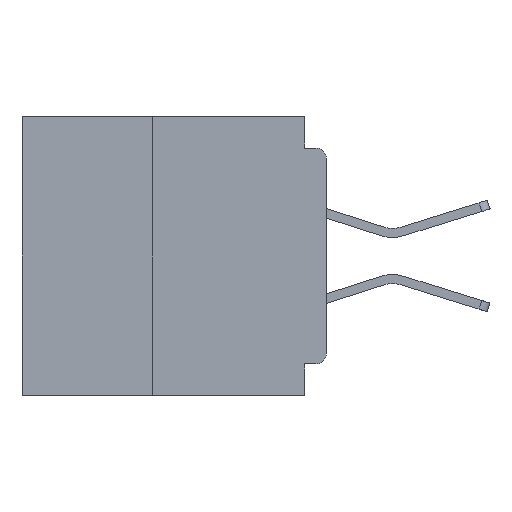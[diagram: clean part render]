
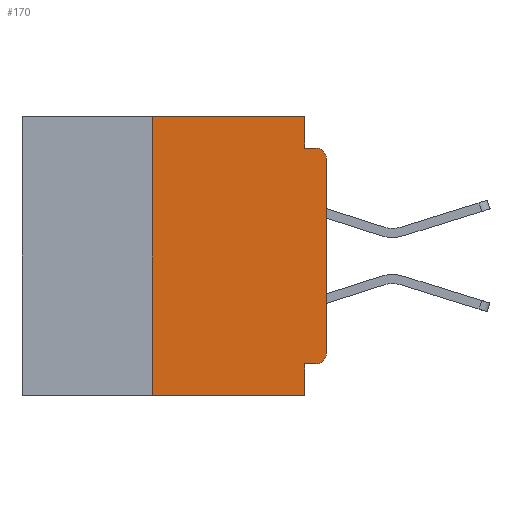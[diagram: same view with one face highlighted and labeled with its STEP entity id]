
A CAD part, left-side view. The second image highlights one B-rep face of the part: STEP entity #170.
In plain terms, the highlighted planar face has unit normal (-1, 0, 0).
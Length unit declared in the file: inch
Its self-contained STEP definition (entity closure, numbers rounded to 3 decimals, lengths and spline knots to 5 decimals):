
#170 = ADVANCED_FACE ( 'NONE', ( #20873 ), #18530, .F. ) ;
#256 = CARTESIAN_POINT ( 'NONE',  ( 0., 0.25, -0.4 ) ) ;
#1623 = CARTESIAN_POINT ( 'NONE',  ( 0., 0., -0.06 ) ) ;
#1699 = VERTEX_POINT ( 'NONE', #38426 ) ;
#2398 = DIRECTION ( 'NONE',  ( 0., 0., -1. ) ) ;
#3183 = CARTESIAN_POINT ( 'NONE',  ( 0., 0., 0. ) ) ;
#3210 = EDGE_CURVE ( 'NONE', #23227, #28093, #6582, .T. ) ;
#4057 = EDGE_CURVE ( 'NONE', #31193, #38917, #17491, .T. ) ;
#4958 = CARTESIAN_POINT ( 'NONE',  ( 0., 0.437, 0. ) ) ;
#5925 = ORIENTED_EDGE ( 'NONE', *, *, #26304, .F. ) ;
#5983 = DIRECTION ( 'NONE',  ( 0., 0., 1. ) ) ;
#6258 = DIRECTION ( 'NONE',  ( 1., 0., 0. ) ) ;
#6339 = CARTESIAN_POINT ( 'NONE',  ( 0., 0.437, 0. ) ) ;
#6582 = LINE ( 'NONE', #3183, #29655 ) ;
#6968 = VECTOR ( 'NONE', #35060, 39.37008 ) ;
#7051 = EDGE_CURVE ( 'NONE', #28093, #1699, #12735, .T. ) ;
#7144 = AXIS2_PLACEMENT_3D ( 'NONE', #6339, #6258, #16620 ) ;
#7480 = DIRECTION ( 'NONE',  ( 0., 0., -1. ) ) ;
#7522 = EDGE_CURVE ( 'NONE', #19861, #24363, #33693, .T. ) ;
#8342 = CARTESIAN_POINT ( 'NONE',  ( 0., 0.25, -0.4 ) ) ;
#9423 = VECTOR ( 'NONE', #36320, 39.37008 ) ;
#10549 = LINE ( 'NONE', #25515, #25561 ) ;
#10840 = CARTESIAN_POINT ( 'NONE',  ( 0., 0.437, -0.4 ) ) ;
#11797 = EDGE_CURVE ( 'NONE', #18014, #23227, #34766, .T. ) ;
#12735 = CIRCLE ( 'NONE', #15233, 0.015 ) ;
#13312 = ORIENTED_EDGE ( 'NONE', *, *, #22354, .F. ) ;
#13706 = ORIENTED_EDGE ( 'NONE', *, *, #3210, .T. ) ;
#13875 = DIRECTION ( 'NONE',  ( -1., 0., 0. ) ) ;
#13972 = LINE ( 'NONE', #25414, #28967 ) ;
#14930 = CARTESIAN_POINT ( 'NONE',  ( 0., 0.25, 0. ) ) ;
#15059 = LINE ( 'NONE', #4958, #6968 ) ;
#15233 = AXIS2_PLACEMENT_3D ( 'NONE', #38491, #20638, #2398 ) ;
#15668 = VECTOR ( 'NONE', #27492, 39.37008 ) ;
#16032 = LINE ( 'NONE', #8342, #30017 ) ;
#16620 = DIRECTION ( 'NONE',  ( 0., 0., -1. ) ) ;
#17491 = LINE ( 'NONE', #36276, #9423 ) ;
#18014 = VERTEX_POINT ( 'NONE', #20208 ) ;
#18530 = PLANE ( 'NONE',  #7144 ) ;
#18863 = VECTOR ( 'NONE', #31731, 39.37008 ) ;
#19861 = VERTEX_POINT ( 'NONE', #256 ) ;
#20208 = CARTESIAN_POINT ( 'NONE',  ( 0., 0.015, -0.355 ) ) ;
#20610 = EDGE_LOOP ( 'NONE', ( #13706, #39123, #5925, #32195, #37987, #13312, #23465, #28019, #34360, #32625 ) ) ;
#20638 = DIRECTION ( 'NONE',  ( -1., 0., 0. ) ) ;
#20873 = FACE_OUTER_BOUND ( 'NONE', #20610, .T. ) ;
#21485 = CARTESIAN_POINT ( 'NONE',  ( 0., 0., -0.045 ) ) ;
#22324 = EDGE_CURVE ( 'NONE', #31907, #31193, #15059, .T. ) ;
#22354 = EDGE_CURVE ( 'NONE', #19861, #31907, #16032, .T. ) ;
#23227 = VERTEX_POINT ( 'NONE', #27350 ) ;
#23465 = ORIENTED_EDGE ( 'NONE', *, *, #7522, .T. ) ;
#23587 = LINE ( 'NONE', #21485, #15668 ) ;
#24363 = VERTEX_POINT ( 'NONE', #32765 ) ;
#25414 = CARTESIAN_POINT ( 'NONE',  ( 0., 0., -0.355 ) ) ;
#25515 = CARTESIAN_POINT ( 'NONE',  ( 0., 0.031, -0.4 ) ) ;
#25561 = VECTOR ( 'NONE', #7480, 39.37008 ) ;
#25778 = CARTESIAN_POINT ( 'NONE',  ( 0., 0.031, -0.355 ) ) ;
#26304 = EDGE_CURVE ( 'NONE', #38917, #1699, #23587, .T. ) ;
#27350 = CARTESIAN_POINT ( 'NONE',  ( 0., 0., -0.34 ) ) ;
#27492 = DIRECTION ( 'NONE',  ( 0., -1., 0. ) ) ;
#28019 = ORIENTED_EDGE ( 'NONE', *, *, #37752, .F. ) ;
#28093 = VERTEX_POINT ( 'NONE', #1623 ) ;
#28422 = DIRECTION ( 'NONE',  ( 0., 1., 0. ) ) ;
#28967 = VECTOR ( 'NONE', #28422, 39.37008 ) ;
#29370 = AXIS2_PLACEMENT_3D ( 'NONE', #31750, #13875, #34764 ) ;
#29655 = VECTOR ( 'NONE', #5983, 39.37008 ) ;
#29796 = CARTESIAN_POINT ( 'NONE',  ( 0., 0.031, -0.045 ) ) ;
#29801 = EDGE_CURVE ( 'NONE', #18014, #37800, #13972, .T. ) ;
#30017 = VECTOR ( 'NONE', #35184, 39.37008 ) ;
#31193 = VERTEX_POINT ( 'NONE', #35490 ) ;
#31731 = DIRECTION ( 'NONE',  ( 0., -1., 0. ) ) ;
#31750 = CARTESIAN_POINT ( 'NONE',  ( 0., 0.015, -0.34 ) ) ;
#31907 = VERTEX_POINT ( 'NONE', #14930 ) ;
#32195 = ORIENTED_EDGE ( 'NONE', *, *, #4057, .F. ) ;
#32625 = ORIENTED_EDGE ( 'NONE', *, *, #11797, .T. ) ;
#32765 = CARTESIAN_POINT ( 'NONE',  ( 0., 0.031, -0.4 ) ) ;
#33693 = LINE ( 'NONE', #10840, #18863 ) ;
#34360 = ORIENTED_EDGE ( 'NONE', *, *, #29801, .F. ) ;
#34764 = DIRECTION ( 'NONE',  ( 0., 0., -1. ) ) ;
#34766 = CIRCLE ( 'NONE', #29370, 0.015 ) ;
#35060 = DIRECTION ( 'NONE',  ( 0., -1., 0. ) ) ;
#35184 = DIRECTION ( 'NONE',  ( 0., 0., 1. ) ) ;
#35490 = CARTESIAN_POINT ( 'NONE',  ( 0., 0.031, 0. ) ) ;
#36276 = CARTESIAN_POINT ( 'NONE',  ( 0., 0.031, 0. ) ) ;
#36320 = DIRECTION ( 'NONE',  ( 0., 0., -1. ) ) ;
#37752 = EDGE_CURVE ( 'NONE', #37800, #24363, #10549, .T. ) ;
#37800 = VERTEX_POINT ( 'NONE', #25778 ) ;
#37987 = ORIENTED_EDGE ( 'NONE', *, *, #22324, .F. ) ;
#38426 = CARTESIAN_POINT ( 'NONE',  ( 0., 0.015, -0.045 ) ) ;
#38491 = CARTESIAN_POINT ( 'NONE',  ( 0., 0.015, -0.06 ) ) ;
#38917 = VERTEX_POINT ( 'NONE', #29796 ) ;
#39123 = ORIENTED_EDGE ( 'NONE', *, *, #7051, .T. ) ;
